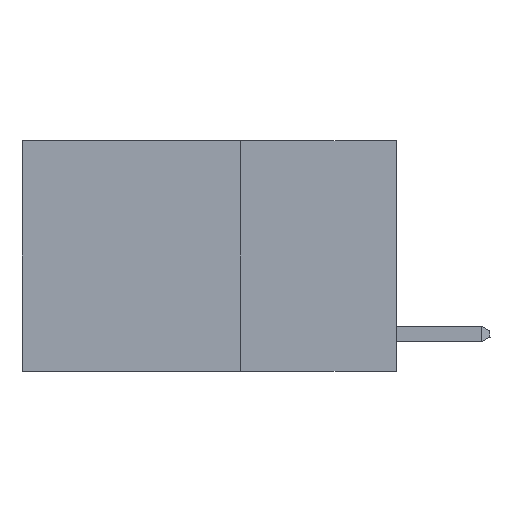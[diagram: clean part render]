
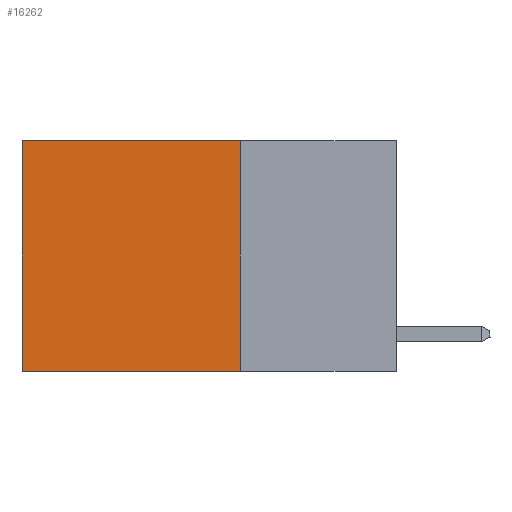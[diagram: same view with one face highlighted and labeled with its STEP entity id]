
A CAD part, left-side view. The second image highlights one B-rep face of the part: STEP entity #16262.
In plain terms, the highlighted planar face has unit normal (-1, 0, 0).
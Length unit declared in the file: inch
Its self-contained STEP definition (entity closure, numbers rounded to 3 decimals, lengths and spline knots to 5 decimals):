
#457 = VECTOR ( 'NONE', #4147, 39.37008 ) ;
#1685 = CARTESIAN_POINT ( 'NONE',  ( 0.2625, 0.25, 0. ) ) ;
#2399 = DIRECTION ( 'NONE',  ( 0., 0., -1. ) ) ;
#3030 = VECTOR ( 'NONE', #3558, 39.37008 ) ;
#3448 = VERTEX_POINT ( 'NONE', #4570 ) ;
#3558 = DIRECTION ( 'NONE',  ( 0., 0., -1. ) ) ;
#3611 = LINE ( 'NONE', #1685, #3030 ) ;
#4147 = DIRECTION ( 'NONE',  ( 0., 1., 0. ) ) ;
#4202 = AXIS2_PLACEMENT_3D ( 'NONE', #17110, #13509, #2399 ) ;
#4570 = CARTESIAN_POINT ( 'NONE',  ( 0.2625, 0.25, -0.37 ) ) ;
#7421 = VECTOR ( 'NONE', #15421, 39.37008 ) ;
#7860 = ORIENTED_EDGE ( 'NONE', *, *, #19164, .T. ) ;
#8943 = ORIENTED_EDGE ( 'NONE', *, *, #19170, .T. ) ;
#9003 = FACE_OUTER_BOUND ( 'NONE', #14312, .T. ) ;
#9466 = VERTEX_POINT ( 'NONE', #9888 ) ;
#9876 = DIRECTION ( 'NONE',  ( 0., 1., 0. ) ) ;
#9888 = CARTESIAN_POINT ( 'NONE',  ( 0.2625, 0.6, 0. ) ) ;
#10016 = CARTESIAN_POINT ( 'NONE',  ( 0.2625, 0.6, -0.37 ) ) ;
#11630 = PLANE ( 'NONE',  #4202 ) ;
#12577 = LINE ( 'NONE', #20769, #22067 ) ;
#13461 = ORIENTED_EDGE ( 'NONE', *, *, #18902, .F. ) ;
#13509 = DIRECTION ( 'NONE',  ( 1., 0., 0. ) ) ;
#13598 = CARTESIAN_POINT ( 'NONE',  ( 0.2625, 0.6, 0. ) ) ;
#13710 = VERTEX_POINT ( 'NONE', #16179 ) ;
#14312 = EDGE_LOOP ( 'NONE', ( #8943, #23561, #13461, #7860 ) ) ;
#15421 = DIRECTION ( 'NONE',  ( 0., 0., -1. ) ) ;
#16179 = CARTESIAN_POINT ( 'NONE',  ( 0.2625, 0.25, 0. ) ) ;
#16262 = ADVANCED_FACE ( 'NONE', ( #9003 ), #11630, .F. ) ;
#17110 = CARTESIAN_POINT ( 'NONE',  ( 0.2625, 0.25, 0. ) ) ;
#17457 = LINE ( 'NONE', #13598, #7421 ) ;
#17930 = VERTEX_POINT ( 'NONE', #10016 ) ;
#18902 = EDGE_CURVE ( 'NONE', #13710, #3448, #3611, .T. ) ;
#19164 = EDGE_CURVE ( 'NONE', #13710, #9466, #12577, .T. ) ;
#19170 = EDGE_CURVE ( 'NONE', #9466, #17930, #17457, .T. ) ;
#19482 = LINE ( 'NONE', #22479, #457 ) ;
#20769 = CARTESIAN_POINT ( 'NONE',  ( 0.2625, 0.25, 0. ) ) ;
#22067 = VECTOR ( 'NONE', #9876, 39.37008 ) ;
#22479 = CARTESIAN_POINT ( 'NONE',  ( 0.2625, 0.25, -0.37 ) ) ;
#23561 = ORIENTED_EDGE ( 'NONE', *, *, #23626, .F. ) ;
#23626 = EDGE_CURVE ( 'NONE', #3448, #17930, #19482, .T. ) ;
